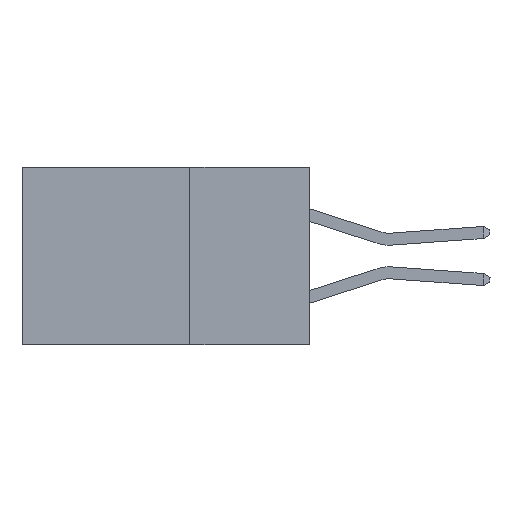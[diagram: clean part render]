
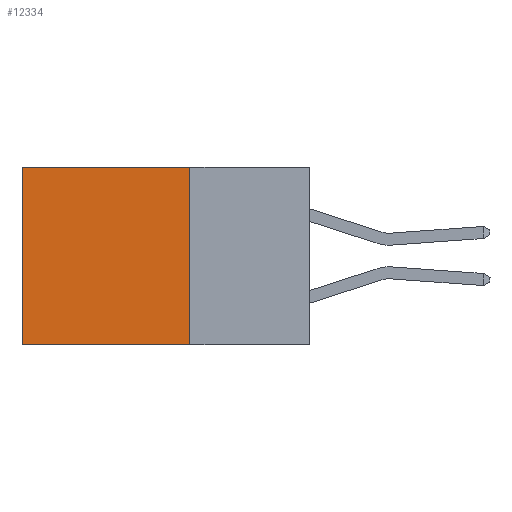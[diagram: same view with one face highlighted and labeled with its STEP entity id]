
A CAD part, left-side view. The second image highlights one B-rep face of the part: STEP entity #12334.
In plain terms, the highlighted planar face has unit normal (-1, 0, 0).
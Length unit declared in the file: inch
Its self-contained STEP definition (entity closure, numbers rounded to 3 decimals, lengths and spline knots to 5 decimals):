
#232 = LINE ( 'NONE', #10845, #15508 ) ;
#436 = DIRECTION ( 'NONE',  ( 0., 0., -1. ) ) ;
#1033 = CARTESIAN_POINT ( 'NONE',  ( 0.298, 0.25, -0.37 ) ) ;
#2050 = PLANE ( 'NONE',  #20887 ) ;
#2179 = ORIENTED_EDGE ( 'NONE', *, *, #18486, .F. ) ;
#3285 = CARTESIAN_POINT ( 'NONE',  ( 0.298, 0.25, 0. ) ) ;
#3868 = ORIENTED_EDGE ( 'NONE', *, *, #9197, .F. ) ;
#4230 = DIRECTION ( 'NONE',  ( 1., 0., 0. ) ) ;
#4809 = VERTEX_POINT ( 'NONE', #1033 ) ;
#8828 = DIRECTION ( 'NONE',  ( 0., 1., 0. ) ) ;
#9197 = EDGE_CURVE ( 'NONE', #21322, #4809, #232, .T. ) ;
#9402 = LINE ( 'NONE', #24560, #25667 ) ;
#9917 = CARTESIAN_POINT ( 'NONE',  ( 0.298, 0.6, 0. ) ) ;
#10845 = CARTESIAN_POINT ( 'NONE',  ( 0.298, 0.25, 0. ) ) ;
#10967 = LINE ( 'NONE', #19663, #16202 ) ;
#12334 = ADVANCED_FACE ( 'NONE', ( #25434 ), #2050, .F. ) ;
#13616 = VERTEX_POINT ( 'NONE', #22981 ) ;
#14192 = EDGE_LOOP ( 'NONE', ( #19462, #2179, #3868, #18203 ) ) ;
#14530 = DIRECTION ( 'NONE',  ( 0., 0., -1. ) ) ;
#15508 = VECTOR ( 'NONE', #436, 39.37008 ) ;
#16202 = VECTOR ( 'NONE', #8828, 39.37008 ) ;
#16349 = DIRECTION ( 'NONE',  ( 0., 0., -1. ) ) ;
#16512 = EDGE_CURVE ( 'NONE', #19829, #13616, #9402, .T. ) ;
#17833 = VECTOR ( 'NONE', #24122, 39.37008 ) ;
#18203 = ORIENTED_EDGE ( 'NONE', *, *, #25407, .T. ) ;
#18486 = EDGE_CURVE ( 'NONE', #4809, #13616, #10967, .T. ) ;
#19462 = ORIENTED_EDGE ( 'NONE', *, *, #16512, .T. ) ;
#19663 = CARTESIAN_POINT ( 'NONE',  ( 0.298, 0.25, -0.37 ) ) ;
#19829 = VERTEX_POINT ( 'NONE', #9917 ) ;
#20887 = AXIS2_PLACEMENT_3D ( 'NONE', #22891, #4230, #14530 ) ;
#21322 = VERTEX_POINT ( 'NONE', #24980 ) ;
#22891 = CARTESIAN_POINT ( 'NONE',  ( 0.298, 0.25, 0. ) ) ;
#22981 = CARTESIAN_POINT ( 'NONE',  ( 0.298, 0.6, -0.37 ) ) ;
#23337 = LINE ( 'NONE', #3285, #17833 ) ;
#24122 = DIRECTION ( 'NONE',  ( 0., 1., 0. ) ) ;
#24560 = CARTESIAN_POINT ( 'NONE',  ( 0.298, 0.6, 0. ) ) ;
#24980 = CARTESIAN_POINT ( 'NONE',  ( 0.298, 0.25, 0. ) ) ;
#25407 = EDGE_CURVE ( 'NONE', #21322, #19829, #23337, .T. ) ;
#25434 = FACE_OUTER_BOUND ( 'NONE', #14192, .T. ) ;
#25667 = VECTOR ( 'NONE', #16349, 39.37008 ) ;
